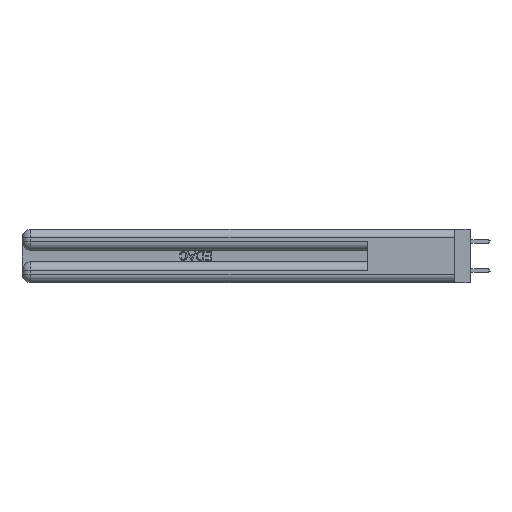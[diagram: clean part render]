
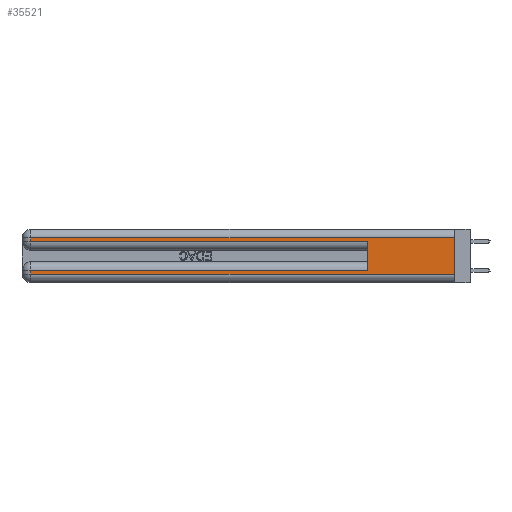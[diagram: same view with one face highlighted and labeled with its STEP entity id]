
A CAD part, left-side view. The second image highlights one B-rep face of the part: STEP entity #35521.
In plain terms, the highlighted planar face has unit normal (-1, 0, 0).
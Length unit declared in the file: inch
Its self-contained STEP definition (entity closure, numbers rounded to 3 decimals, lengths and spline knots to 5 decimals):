
#188 = ORIENTED_EDGE ( 'NONE', *, *, #41475, .F. ) ;
#453 = VECTOR ( 'NONE', #34810, 39.37008 ) ;
#655 = VERTEX_POINT ( 'NONE', #27160 ) ;
#809 = VECTOR ( 'NONE', #19351, 39.37008 ) ;
#1173 = CARTESIAN_POINT ( 'NONE',  ( 0., 2.94, 0.37 ) ) ;
#1972 = CARTESIAN_POINT ( 'NONE',  ( 0., 0.6, 0.285 ) ) ;
#2442 = DIRECTION ( 'NONE',  ( 1., 0., 0. ) ) ;
#2477 = DIRECTION ( 'NONE',  ( 0., -1., 0. ) ) ;
#2529 = CARTESIAN_POINT ( 'NONE',  ( 0., 0., 0.06 ) ) ;
#2838 = ORIENTED_EDGE ( 'NONE', *, *, #15020, .F. ) ;
#6324 = LINE ( 'NONE', #25923, #15306 ) ;
#6378 = VECTOR ( 'NONE', #20260, 39.37008 ) ;
#6744 = ORIENTED_EDGE ( 'NONE', *, *, #17574, .T. ) ;
#8005 = AXIS2_PLACEMENT_3D ( 'NONE', #12496, #2442, #26159 ) ;
#8395 = LINE ( 'NONE', #1173, #453 ) ;
#8701 = CARTESIAN_POINT ( 'NONE',  ( 0., 0., 0.285 ) ) ;
#9011 = DIRECTION ( 'NONE',  ( 0., 1., 0. ) ) ;
#11872 = EDGE_CURVE ( 'NONE', #35775, #37725, #6324, .T. ) ;
#12496 = CARTESIAN_POINT ( 'NONE',  ( 0., 0., 0.37 ) ) ;
#13537 = CARTESIAN_POINT ( 'NONE',  ( 0., 2.94, 0.31 ) ) ;
#13967 = CARTESIAN_POINT ( 'NONE',  ( 0., 0.6, 0.085 ) ) ;
#14916 = VECTOR ( 'NONE', #38486, 39.37008 ) ;
#14960 = CARTESIAN_POINT ( 'NONE',  ( 0., 0., 0.31 ) ) ;
#15020 = EDGE_CURVE ( 'NONE', #29698, #36219, #30962, .T. ) ;
#15306 = VECTOR ( 'NONE', #9011, 39.37008 ) ;
#16394 = CARTESIAN_POINT ( 'NONE',  ( 0., 0., 0.31 ) ) ;
#17574 = EDGE_CURVE ( 'NONE', #29698, #31702, #32852, .T. ) ;
#19351 = DIRECTION ( 'NONE',  ( 0., 0., -1. ) ) ;
#20021 = ORIENTED_EDGE ( 'NONE', *, *, #36654, .T. ) ;
#20260 = DIRECTION ( 'NONE',  ( 0., 0., 1. ) ) ;
#20413 = CARTESIAN_POINT ( 'NONE',  ( 0., 0.6, 0.145 ) ) ;
#20932 = ORIENTED_EDGE ( 'NONE', *, *, #11872, .T. ) ;
#21239 = VERTEX_POINT ( 'NONE', #25782 ) ;
#22674 = VECTOR ( 'NONE', #2477, 39.37008 ) ;
#25782 = CARTESIAN_POINT ( 'NONE',  ( 0., 2.94, 0.06 ) ) ;
#25923 = CARTESIAN_POINT ( 'NONE',  ( 0., 0., 0.085 ) ) ;
#26159 = DIRECTION ( 'NONE',  ( 0., 0., -1. ) ) ;
#27160 = CARTESIAN_POINT ( 'NONE',  ( 0., 2.94, 0.285 ) ) ;
#27738 = EDGE_LOOP ( 'NONE', ( #2838, #6744, #20021, #40615, #188, #20932, #30576, #35407 ) ) ;
#29036 = LINE ( 'NONE', #8701, #37867 ) ;
#29521 = EDGE_CURVE ( 'NONE', #655, #32055, #29036, .T. ) ;
#29698 = VERTEX_POINT ( 'NONE', #16394 ) ;
#30440 = LINE ( 'NONE', #37986, #38268 ) ;
#30576 = ORIENTED_EDGE ( 'NONE', *, *, #38365, .T. ) ;
#30962 = LINE ( 'NONE', #42687, #809 ) ;
#31702 = VERTEX_POINT ( 'NONE', #13537 ) ;
#32055 = VERTEX_POINT ( 'NONE', #1972 ) ;
#32241 = LINE ( 'NONE', #20413, #6378 ) ;
#32717 = PLANE ( 'NONE',  #8005 ) ;
#32852 = LINE ( 'NONE', #14960, #14916 ) ;
#34810 = DIRECTION ( 'NONE',  ( 0., 0., -1. ) ) ;
#35407 = ORIENTED_EDGE ( 'NONE', *, *, #36940, .T. ) ;
#35521 = ADVANCED_FACE ( 'NONE', ( #35853 ), #32717, .F. ) ;
#35660 = DIRECTION ( 'NONE',  ( 0., -1., 0. ) ) ;
#35775 = VERTEX_POINT ( 'NONE', #13967 ) ;
#35853 = FACE_OUTER_BOUND ( 'NONE', #27738, .T. ) ;
#36219 = VERTEX_POINT ( 'NONE', #2529 ) ;
#36654 = EDGE_CURVE ( 'NONE', #31702, #655, #8395, .T. ) ;
#36940 = EDGE_CURVE ( 'NONE', #21239, #36219, #40452, .T. ) ;
#37725 = VERTEX_POINT ( 'NONE', #38232 ) ;
#37867 = VECTOR ( 'NONE', #35660, 39.37008 ) ;
#37986 = CARTESIAN_POINT ( 'NONE',  ( 0., 2.94, 0.37 ) ) ;
#38232 = CARTESIAN_POINT ( 'NONE',  ( 0., 2.94, 0.085 ) ) ;
#38268 = VECTOR ( 'NONE', #41317, 39.37008 ) ;
#38365 = EDGE_CURVE ( 'NONE', #37725, #21239, #30440, .T. ) ;
#38486 = DIRECTION ( 'NONE',  ( 0., 1., 0. ) ) ;
#40452 = LINE ( 'NONE', #42745, #22674 ) ;
#40615 = ORIENTED_EDGE ( 'NONE', *, *, #29521, .T. ) ;
#41317 = DIRECTION ( 'NONE',  ( 0., 0., -1. ) ) ;
#41475 = EDGE_CURVE ( 'NONE', #35775, #32055, #32241, .T. ) ;
#42687 = CARTESIAN_POINT ( 'NONE',  ( 0., 0., 0.37 ) ) ;
#42745 = CARTESIAN_POINT ( 'NONE',  ( 0., 0., 0.06 ) ) ;
